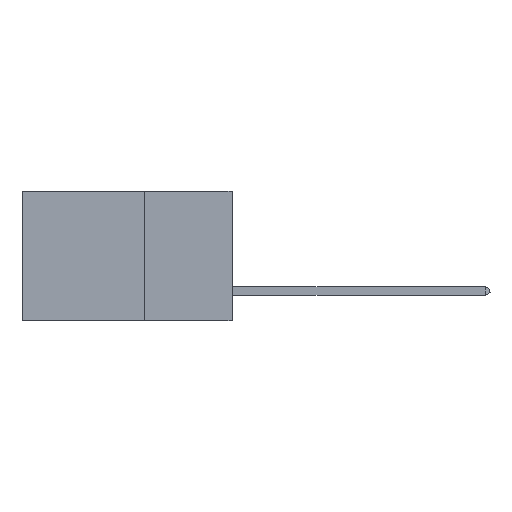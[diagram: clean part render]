
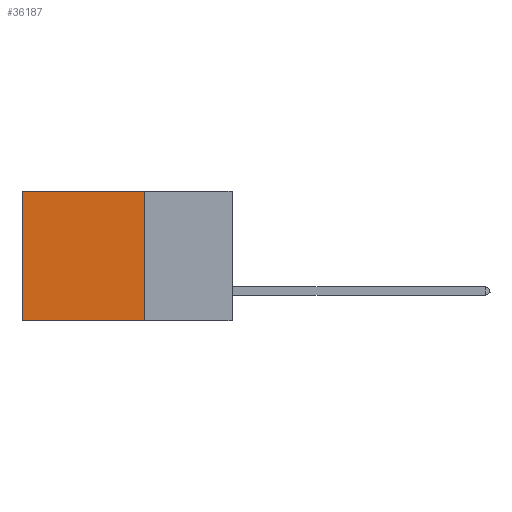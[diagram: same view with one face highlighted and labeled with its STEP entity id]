
A CAD part, left-side view. The second image highlights one B-rep face of the part: STEP entity #36187.
In plain terms, the highlighted planar face has unit normal (-1, 0, 0).
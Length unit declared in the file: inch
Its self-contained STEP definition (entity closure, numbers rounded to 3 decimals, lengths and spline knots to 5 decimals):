
#931 = CARTESIAN_POINT ( 'NONE',  ( 0.2875, 0.6, 0. ) ) ;
#1417 = LINE ( 'NONE', #23371, #42233 ) ;
#2096 = DIRECTION ( 'NONE',  ( 0., 1., 0. ) ) ;
#2275 = PLANE ( 'NONE',  #3859 ) ;
#3859 = AXIS2_PLACEMENT_3D ( 'NONE', #39474, #9373, #29975 ) ;
#5062 = DIRECTION ( 'NONE',  ( 0., 0., -1. ) ) ;
#8987 = FACE_OUTER_BOUND ( 'NONE', #43225, .T. ) ;
#9373 = DIRECTION ( 'NONE',  ( 1., 0., 0. ) ) ;
#10695 = LINE ( 'NONE', #14949, #34578 ) ;
#12190 = EDGE_CURVE ( 'NONE', #42451, #25643, #10695, .T. ) ;
#13660 = VECTOR ( 'NONE', #5062, 39.37008 ) ;
#14515 = DIRECTION ( 'NONE',  ( 0., 1., 0. ) ) ;
#14530 = CARTESIAN_POINT ( 'NONE',  ( 0.2875, 0.6, -0.37 ) ) ;
#14949 = CARTESIAN_POINT ( 'NONE',  ( 0.2875, 0.25, 0. ) ) ;
#15233 = LINE ( 'NONE', #32310, #13660 ) ;
#16013 = ORIENTED_EDGE ( 'NONE', *, *, #22073, .T. ) ;
#16175 = VERTEX_POINT ( 'NONE', #14530 ) ;
#17916 = ORIENTED_EDGE ( 'NONE', *, *, #43506, .F. ) ;
#18788 = CARTESIAN_POINT ( 'NONE',  ( 0.2875, 0.25, -0.37 ) ) ;
#19008 = ORIENTED_EDGE ( 'NONE', *, *, #28334, .F. ) ;
#22073 = EDGE_CURVE ( 'NONE', #25643, #16175, #15233, .T. ) ;
#23371 = CARTESIAN_POINT ( 'NONE',  ( 0.2875, 0.25, 0. ) ) ;
#23519 = DIRECTION ( 'NONE',  ( 0., 0., -1. ) ) ;
#23645 = CARTESIAN_POINT ( 'NONE',  ( 0.2875, 0.25, 0. ) ) ;
#25281 = LINE ( 'NONE', #18788, #32197 ) ;
#25643 = VERTEX_POINT ( 'NONE', #931 ) ;
#26729 = CARTESIAN_POINT ( 'NONE',  ( 0.2875, 0.25, -0.37 ) ) ;
#28334 = EDGE_CURVE ( 'NONE', #42451, #40940, #1417, .T. ) ;
#29975 = DIRECTION ( 'NONE',  ( 0., 0., -1. ) ) ;
#32197 = VECTOR ( 'NONE', #2096, 39.37008 ) ;
#32310 = CARTESIAN_POINT ( 'NONE',  ( 0.2875, 0.6, 0. ) ) ;
#32460 = ORIENTED_EDGE ( 'NONE', *, *, #12190, .T. ) ;
#34578 = VECTOR ( 'NONE', #14515, 39.37008 ) ;
#36187 = ADVANCED_FACE ( 'NONE', ( #8987 ), #2275, .F. ) ;
#39474 = CARTESIAN_POINT ( 'NONE',  ( 0.2875, 0.25, 0. ) ) ;
#40940 = VERTEX_POINT ( 'NONE', #26729 ) ;
#42233 = VECTOR ( 'NONE', #23519, 39.37008 ) ;
#42451 = VERTEX_POINT ( 'NONE', #23645 ) ;
#43225 = EDGE_LOOP ( 'NONE', ( #16013, #17916, #19008, #32460 ) ) ;
#43506 = EDGE_CURVE ( 'NONE', #40940, #16175, #25281, .T. ) ;
